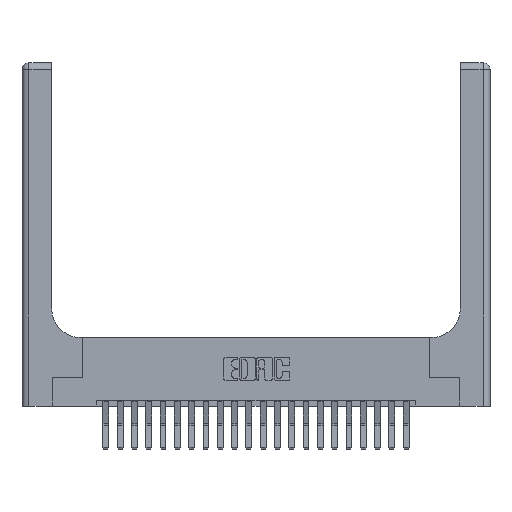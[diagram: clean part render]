
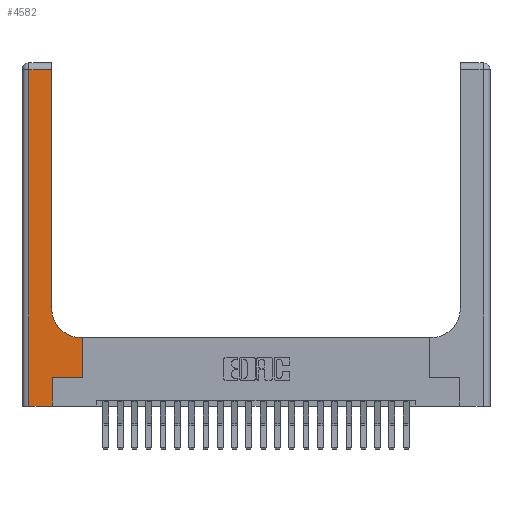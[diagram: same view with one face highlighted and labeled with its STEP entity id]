
A CAD part, top view. The second image highlights one B-rep face of the part: STEP entity #4582.
In plain terms, the highlighted planar face has unit normal (0, 0, 1).
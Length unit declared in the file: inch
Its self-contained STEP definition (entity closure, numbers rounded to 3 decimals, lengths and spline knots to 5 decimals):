
#383 = DIRECTION ( 'NONE',  ( 0., 1., 0. ) ) ;
#633 = LINE ( 'NONE', #19903, #9051 ) ;
#902 = CARTESIAN_POINT ( 'NONE',  ( 0.06, 0., 0.37 ) ) ;
#994 = CARTESIAN_POINT ( 'NONE',  ( 0.265, 0., 0.37 ) ) ;
#1206 = EDGE_CURVE ( 'NONE', #9676, #5328, #10958, .T. ) ;
#2303 = DIRECTION ( 'NONE',  ( 1., 0., 0. ) ) ;
#2370 = CARTESIAN_POINT ( 'NONE',  ( 0.06, 2.94, 0.37 ) ) ;
#3059 = VERTEX_POINT ( 'NONE', #2370 ) ;
#3628 = CARTESIAN_POINT ( 'NONE',  ( 0.265, 0.25, 0.37 ) ) ;
#3838 = CARTESIAN_POINT ( 'NONE',  ( 0.528, 0.25, 0.37 ) ) ;
#4379 = EDGE_CURVE ( 'NONE', #9572, #3059, #633, .T. ) ;
#4479 = LINE ( 'NONE', #5982, #18610 ) ;
#4582 = ADVANCED_FACE ( 'NONE', ( #11737 ), #20406, .F. ) ;
#4688 = VERTEX_POINT ( 'NONE', #17050 ) ;
#4750 = EDGE_CURVE ( 'NONE', #3059, #20290, #4479, .T. ) ;
#5008 = AXIS2_PLACEMENT_3D ( 'NONE', #9904, #17282, #15323 ) ;
#5221 = VECTOR ( 'NONE', #22728, 39.37008 ) ;
#5237 = CARTESIAN_POINT ( 'NONE',  ( 0.265, 0.25, 0.37 ) ) ;
#5328 = VERTEX_POINT ( 'NONE', #10184 ) ;
#5488 = LINE ( 'NONE', #16188, #13189 ) ;
#5535 = VERTEX_POINT ( 'NONE', #9263 ) ;
#5982 = CARTESIAN_POINT ( 'NONE',  ( 0.06, 3., 0.37 ) ) ;
#6124 = CARTESIAN_POINT ( 'NONE',  ( 0.528, 0.25, 0.37 ) ) ;
#7543 = VERTEX_POINT ( 'NONE', #19144 ) ;
#7908 = EDGE_CURVE ( 'NONE', #5328, #7543, #19537, .T. ) ;
#7960 = EDGE_CURVE ( 'NONE', #4688, #9572, #5488, .T. ) ;
#8046 = DIRECTION ( 'NONE',  ( 0., 1., 0. ) ) ;
#8483 = ORIENTED_EDGE ( 'NONE', *, *, #4379, .T. ) ;
#9051 = VECTOR ( 'NONE', #14697, 39.37008 ) ;
#9263 = CARTESIAN_POINT ( 'NONE',  ( 0.265, 0., 0.37 ) ) ;
#9572 = VERTEX_POINT ( 'NONE', #15608 ) ;
#9604 = VECTOR ( 'NONE', #8046, 39.37008 ) ;
#9676 = VERTEX_POINT ( 'NONE', #3838 ) ;
#9904 = CARTESIAN_POINT ( 'NONE',  ( 0., 3., 0.37 ) ) ;
#10184 = CARTESIAN_POINT ( 'NONE',  ( 0.528, 0.6, 0.37 ) ) ;
#10371 = LINE ( 'NONE', #17396, #17399 ) ;
#10958 = LINE ( 'NONE', #6124, #13417 ) ;
#11162 = ORIENTED_EDGE ( 'NONE', *, *, #7960, .T. ) ;
#11195 = ORIENTED_EDGE ( 'NONE', *, *, #20953, .T. ) ;
#11487 = DIRECTION ( 'NONE',  ( 0., -1., 0. ) ) ;
#11713 = VECTOR ( 'NONE', #15849, 39.37008 ) ;
#11737 = FACE_OUTER_BOUND ( 'NONE', #22205, .T. ) ;
#12102 = DIRECTION ( 'NONE',  ( 0., 0., -1. ) ) ;
#13189 = VECTOR ( 'NONE', #383, 39.37008 ) ;
#13417 = VECTOR ( 'NONE', #19953, 39.37008 ) ;
#13444 = AXIS2_PLACEMENT_3D ( 'NONE', #20877, #12102, #2303 ) ;
#14697 = DIRECTION ( 'NONE',  ( -1., 0., 0. ) ) ;
#15323 = DIRECTION ( 'NONE',  ( -1., 0., 0. ) ) ;
#15608 = CARTESIAN_POINT ( 'NONE',  ( 0.26, 2.94, 0.37 ) ) ;
#15849 = DIRECTION ( 'NONE',  ( -1., 0., 0. ) ) ;
#16188 = CARTESIAN_POINT ( 'NONE',  ( 0.26, 3., 0.37 ) ) ;
#16597 = ORIENTED_EDGE ( 'NONE', *, *, #7908, .T. ) ;
#17050 = CARTESIAN_POINT ( 'NONE',  ( 0.26, 0.85, 0.37 ) ) ;
#17282 = DIRECTION ( 'NONE',  ( 0., 0., -1. ) ) ;
#17396 = CARTESIAN_POINT ( 'NONE',  ( 0., 0., 0.37 ) ) ;
#17399 = VECTOR ( 'NONE', #22132, 39.37008 ) ;
#17571 = CARTESIAN_POINT ( 'NONE',  ( 0.26, 0.6, 0.37 ) ) ;
#17938 = ORIENTED_EDGE ( 'NONE', *, *, #18227, .T. ) ;
#18227 = EDGE_CURVE ( 'NONE', #22636, #9676, #20667, .T. ) ;
#18610 = VECTOR ( 'NONE', #11487, 39.37008 ) ;
#19066 = ORIENTED_EDGE ( 'NONE', *, *, #19997, .T. ) ;
#19144 = CARTESIAN_POINT ( 'NONE',  ( 0.51, 0.6, 0.37 ) ) ;
#19497 = ORIENTED_EDGE ( 'NONE', *, *, #21644, .T. ) ;
#19537 = LINE ( 'NONE', #17571, #11713 ) ;
#19555 = ORIENTED_EDGE ( 'NONE', *, *, #4750, .T. ) ;
#19903 = CARTESIAN_POINT ( 'NONE',  ( 0., 2.94, 0.37 ) ) ;
#19953 = DIRECTION ( 'NONE',  ( 0., 1., 0. ) ) ;
#19997 = EDGE_CURVE ( 'NONE', #7543, #4688, #20834, .T. ) ;
#20147 = ORIENTED_EDGE ( 'NONE', *, *, #1206, .T. ) ;
#20290 = VERTEX_POINT ( 'NONE', #902 ) ;
#20406 = PLANE ( 'NONE',  #5008 ) ;
#20667 = LINE ( 'NONE', #5237, #5221 ) ;
#20834 = CIRCLE ( 'NONE', #13444, 0.25 ) ;
#20877 = CARTESIAN_POINT ( 'NONE',  ( 0.51, 0.85, 0.37 ) ) ;
#20953 = EDGE_CURVE ( 'NONE', #5535, #22636, #21984, .T. ) ;
#21644 = EDGE_CURVE ( 'NONE', #20290, #5535, #10371, .T. ) ;
#21984 = LINE ( 'NONE', #994, #9604 ) ;
#22132 = DIRECTION ( 'NONE',  ( 1., 0., 0. ) ) ;
#22205 = EDGE_LOOP ( 'NONE', ( #11162, #8483, #19555, #19497, #11195, #17938, #20147, #16597, #19066 ) ) ;
#22636 = VERTEX_POINT ( 'NONE', #3628 ) ;
#22728 = DIRECTION ( 'NONE',  ( 1., 0., 0. ) ) ;
